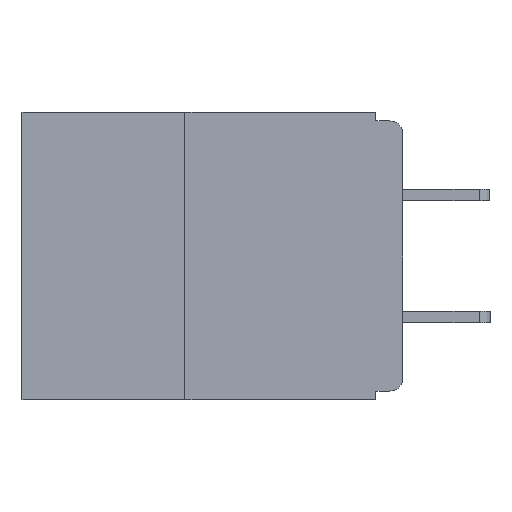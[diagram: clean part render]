
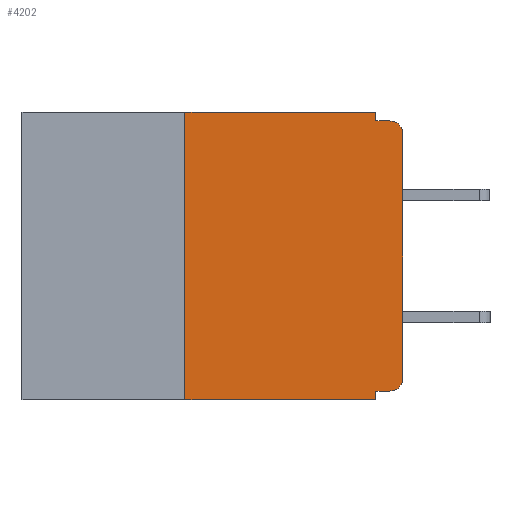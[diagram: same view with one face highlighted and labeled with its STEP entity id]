
A CAD part, left-side view. The second image highlights one B-rep face of the part: STEP entity #4202.
In plain terms, the highlighted planar face has unit normal (-1, 0, 0).
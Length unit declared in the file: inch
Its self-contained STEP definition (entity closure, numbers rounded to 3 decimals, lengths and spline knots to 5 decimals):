
#123 = DIRECTION ( 'NONE',  ( 0., 0., -1. ) ) ;
#128 = DIRECTION ( 'NONE',  ( -1., 0., 0. ) ) ;
#165 = CARTESIAN_POINT ( 'NONE',  ( 0., 0.015, -0.305 ) ) ;
#185 = CARTESIAN_POINT ( 'NONE',  ( 0., 0.031, 0. ) ) ;
#262 = VERTEX_POINT ( 'NONE', #4514 ) ;
#619 = CARTESIAN_POINT ( 'NONE',  ( 0., 0.015, -0.025 ) ) ;
#1005 = DIRECTION ( 'NONE',  ( -1., 0., 0. ) ) ;
#1199 = ORIENTED_EDGE ( 'NONE', *, *, #8669, .F. ) ;
#1676 = EDGE_CURVE ( 'NONE', #7205, #4799, #6791, .T. ) ;
#1714 = CIRCLE ( 'NONE', #12955, 0.015 ) ;
#1733 = DIRECTION ( 'NONE',  ( 0., 0., -1. ) ) ;
#1924 = VECTOR ( 'NONE', #6885, 39.37008 ) ;
#2003 = LINE ( 'NONE', #6712, #1924 ) ;
#2026 = LINE ( 'NONE', #7661, #2083 ) ;
#2083 = VECTOR ( 'NONE', #9225, 39.37008 ) ;
#2199 = ORIENTED_EDGE ( 'NONE', *, *, #4121, .T. ) ;
#2415 = CARTESIAN_POINT ( 'NONE',  ( 0., 0.031, -0.01 ) ) ;
#2917 = ORIENTED_EDGE ( 'NONE', *, *, #7971, .F. ) ;
#3315 = VERTEX_POINT ( 'NONE', #10865 ) ;
#3338 = AXIS2_PLACEMENT_3D ( 'NONE', #165, #128, #123 ) ;
#3346 = CARTESIAN_POINT ( 'NONE',  ( 0., 0., -0.32 ) ) ;
#3476 = DIRECTION ( 'NONE',  ( 0., 1., 0. ) ) ;
#3485 = VERTEX_POINT ( 'NONE', #8727 ) ;
#3509 = CARTESIAN_POINT ( 'NONE',  ( 0., 0.031, -0.32 ) ) ;
#3602 = DIRECTION ( 'NONE',  ( 0., 0., 1. ) ) ;
#3876 = CARTESIAN_POINT ( 'NONE',  ( 0., 0.25, -0.33 ) ) ;
#4121 = EDGE_CURVE ( 'NONE', #7721, #262, #9607, .T. ) ;
#4202 = ADVANCED_FACE ( 'NONE', ( #9213 ), #12889, .F. ) ;
#4473 = EDGE_LOOP ( 'NONE', ( #7137, #11497, #6804, #2917, #8036, #7851, #10365, #9372, #1199, #2199 ) ) ;
#4507 = EDGE_CURVE ( 'NONE', #10780, #11322, #8671, .T. ) ;
#4514 = CARTESIAN_POINT ( 'NONE',  ( 0., 0., -0.305 ) ) ;
#4594 = VECTOR ( 'NONE', #9302, 39.37008 ) ;
#4609 = VECTOR ( 'NONE', #3602, 39.37008 ) ;
#4661 = CARTESIAN_POINT ( 'NONE',  ( 0., 0.015, -0.32 ) ) ;
#4744 = DIRECTION ( 'NONE',  ( 0., -1., 0. ) ) ;
#4799 = VERTEX_POINT ( 'NONE', #5284 ) ;
#4858 = LINE ( 'NONE', #3876, #4609 ) ;
#4977 = DIRECTION ( 'NONE',  ( 0., 0., -1. ) ) ;
#5123 = VECTOR ( 'NONE', #4744, 39.37008 ) ;
#5139 = LINE ( 'NONE', #5563, #5123 ) ;
#5193 = CARTESIAN_POINT ( 'NONE',  ( 0., 0.031, -0.33 ) ) ;
#5284 = CARTESIAN_POINT ( 'NONE',  ( 0., 0.031, -0.33 ) ) ;
#5505 = CARTESIAN_POINT ( 'NONE',  ( 0., 0.015, -0.01 ) ) ;
#5563 = CARTESIAN_POINT ( 'NONE',  ( 0., 0.437, 0. ) ) ;
#5624 = LINE ( 'NONE', #185, #4594 ) ;
#5913 = EDGE_CURVE ( 'NONE', #3315, #6729, #5139, .T. ) ;
#6349 = LINE ( 'NONE', #3346, #8241 ) ;
#6410 = CARTESIAN_POINT ( 'NONE',  ( 0., 0.031, 0. ) ) ;
#6440 = DIRECTION ( 'NONE',  ( 0., -1., 0. ) ) ;
#6712 = CARTESIAN_POINT ( 'NONE',  ( 0., 0., 0. ) ) ;
#6729 = VERTEX_POINT ( 'NONE', #6410 ) ;
#6791 = LINE ( 'NONE', #5193, #6833 ) ;
#6804 = ORIENTED_EDGE ( 'NONE', *, *, #4507, .F. ) ;
#6833 = VECTOR ( 'NONE', #4977, 39.37008 ) ;
#6885 = DIRECTION ( 'NONE',  ( 0., 0., 1. ) ) ;
#7066 = CARTESIAN_POINT ( 'NONE',  ( 0., 0., -0.01 ) ) ;
#7133 = EDGE_CURVE ( 'NONE', #3485, #4799, #2026, .T. ) ;
#7137 = ORIENTED_EDGE ( 'NONE', *, *, #7150, .T. ) ;
#7150 = EDGE_CURVE ( 'NONE', #262, #13048, #2003, .T. ) ;
#7205 = VERTEX_POINT ( 'NONE', #3509 ) ;
#7235 = EDGE_CURVE ( 'NONE', #13048, #11322, #1714, .T. ) ;
#7481 = CARTESIAN_POINT ( 'NONE',  ( 0., 0., -0.025 ) ) ;
#7661 = CARTESIAN_POINT ( 'NONE',  ( 0., 0.437, -0.33 ) ) ;
#7721 = VERTEX_POINT ( 'NONE', #4661 ) ;
#7851 = ORIENTED_EDGE ( 'NONE', *, *, #10065, .F. ) ;
#7971 = EDGE_CURVE ( 'NONE', #6729, #10780, #5624, .T. ) ;
#8036 = ORIENTED_EDGE ( 'NONE', *, *, #5913, .F. ) ;
#8241 = VECTOR ( 'NONE', #3476, 39.37008 ) ;
#8661 = VECTOR ( 'NONE', #6440, 39.37008 ) ;
#8669 = EDGE_CURVE ( 'NONE', #7721, #7205, #6349, .T. ) ;
#8671 = LINE ( 'NONE', #7066, #8661 ) ;
#8727 = CARTESIAN_POINT ( 'NONE',  ( 0., 0.25, -0.33 ) ) ;
#9213 = FACE_OUTER_BOUND ( 'NONE', #4473, .T. ) ;
#9225 = DIRECTION ( 'NONE',  ( 0., -1., 0. ) ) ;
#9302 = DIRECTION ( 'NONE',  ( 0., 0., -1. ) ) ;
#9372 = ORIENTED_EDGE ( 'NONE', *, *, #1676, .F. ) ;
#9607 = CIRCLE ( 'NONE', #3338, 0.015 ) ;
#10065 = EDGE_CURVE ( 'NONE', #3485, #3315, #4858, .T. ) ;
#10365 = ORIENTED_EDGE ( 'NONE', *, *, #7133, .T. ) ;
#10780 = VERTEX_POINT ( 'NONE', #2415 ) ;
#10865 = CARTESIAN_POINT ( 'NONE',  ( 0., 0.25, 0. ) ) ;
#11322 = VERTEX_POINT ( 'NONE', #5505 ) ;
#11497 = ORIENTED_EDGE ( 'NONE', *, *, #7235, .T. ) ;
#12505 = DIRECTION ( 'NONE',  ( 0., 0., -1. ) ) ;
#12612 = DIRECTION ( 'NONE',  ( 1., 0., 0. ) ) ;
#12855 = AXIS2_PLACEMENT_3D ( 'NONE', #13123, #12612, #12505 ) ;
#12889 = PLANE ( 'NONE',  #12855 ) ;
#12955 = AXIS2_PLACEMENT_3D ( 'NONE', #619, #1005, #1733 ) ;
#13048 = VERTEX_POINT ( 'NONE', #7481 ) ;
#13123 = CARTESIAN_POINT ( 'NONE',  ( 0., 0.437, 0. ) ) ;
